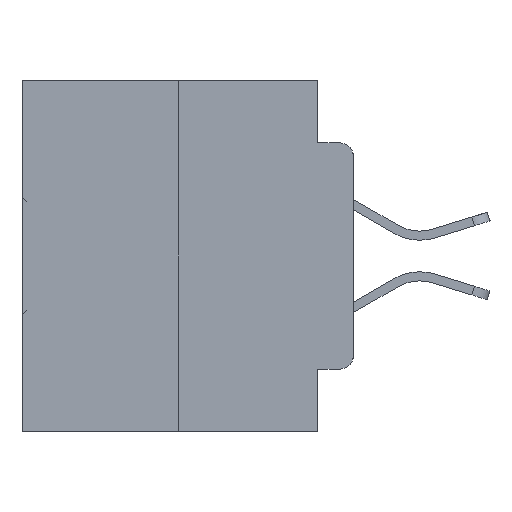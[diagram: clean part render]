
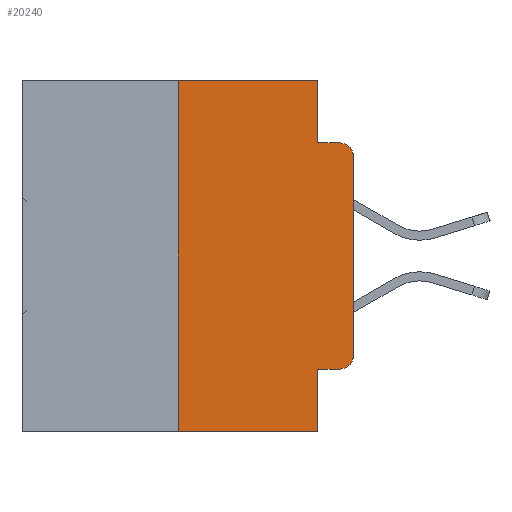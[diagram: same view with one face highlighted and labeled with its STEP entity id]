
A CAD part, left-side view. The second image highlights one B-rep face of the part: STEP entity #20240.
In plain terms, the highlighted planar face has unit normal (-1, 0, 0).
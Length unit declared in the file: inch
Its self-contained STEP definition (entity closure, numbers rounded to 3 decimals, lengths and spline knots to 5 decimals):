
#207 = EDGE_CURVE ( 'NONE', #18751, #5665, #8600, .T. ) ;
#492 = CARTESIAN_POINT ( 'NONE',  ( 0., 0.051, 0. ) ) ;
#687 = CARTESIAN_POINT ( 'NONE',  ( 0., 0.02, -0.4115 ) ) ;
#1872 = CARTESIAN_POINT ( 'NONE',  ( 0., 0.051, 0. ) ) ;
#2226 = CARTESIAN_POINT ( 'NONE',  ( 0., 0.051, -0.5 ) ) ;
#2351 = LINE ( 'NONE', #10271, #21443 ) ;
#2475 = CARTESIAN_POINT ( 'NONE',  ( 0., 0.473, -0.5 ) ) ;
#2622 = AXIS2_PLACEMENT_3D ( 'NONE', #25559, #23217, #22885 ) ;
#2670 = FACE_OUTER_BOUND ( 'NONE', #24543, .T. ) ;
#3357 = ORIENTED_EDGE ( 'NONE', *, *, #25172, .T. ) ;
#3578 = CARTESIAN_POINT ( 'NONE',  ( 0., 0.02, -0.0885 ) ) ;
#4313 = VERTEX_POINT ( 'NONE', #28794 ) ;
#4670 = LINE ( 'NONE', #2475, #7825 ) ;
#4744 = DIRECTION ( 'NONE',  ( 0., 0., -1. ) ) ;
#5144 = VECTOR ( 'NONE', #4744, 39.37008 ) ;
#5547 = ORIENTED_EDGE ( 'NONE', *, *, #18010, .F. ) ;
#5665 = VERTEX_POINT ( 'NONE', #19399 ) ;
#6133 = ORIENTED_EDGE ( 'NONE', *, *, #15103, .F. ) ;
#7130 = DIRECTION ( 'NONE',  ( 0., 0., 1. ) ) ;
#7234 = EDGE_CURVE ( 'NONE', #31207, #4313, #7448, .T. ) ;
#7403 = ORIENTED_EDGE ( 'NONE', *, *, #30107, .T. ) ;
#7448 = CIRCLE ( 'NONE', #13898, 0.02 ) ;
#7552 = DIRECTION ( 'NONE',  ( 0., -1., 0. ) ) ;
#7616 = LINE ( 'NONE', #1872, #5144 ) ;
#7628 = LINE ( 'NONE', #18245, #24825 ) ;
#7746 = EDGE_CURVE ( 'NONE', #26955, #31207, #24942, .T. ) ;
#7825 = VECTOR ( 'NONE', #7552, 39.37008 ) ;
#8117 = DIRECTION ( 'NONE',  ( 0., 0., -1. ) ) ;
#8600 = LINE ( 'NONE', #492, #26900 ) ;
#10271 = CARTESIAN_POINT ( 'NONE',  ( 0., 0.473, 0. ) ) ;
#11434 = VECTOR ( 'NONE', #11779, 39.37008 ) ;
#11779 = DIRECTION ( 'NONE',  ( 0., -1., 0. ) ) ;
#11863 = ORIENTED_EDGE ( 'NONE', *, *, #27198, .F. ) ;
#12675 = DIRECTION ( 'NONE',  ( -1., 0., 0. ) ) ;
#13898 = AXIS2_PLACEMENT_3D ( 'NONE', #17749, #12675, #8117 ) ;
#14205 = CARTESIAN_POINT ( 'NONE',  ( 0., 0.051, 0. ) ) ;
#14798 = CIRCLE ( 'NONE', #22863, 0.02 ) ;
#14809 = CARTESIAN_POINT ( 'NONE',  ( 0., 0.051, -0.0885 ) ) ;
#15103 = EDGE_CURVE ( 'NONE', #26955, #24203, #7616, .T. ) ;
#16980 = VERTEX_POINT ( 'NONE', #22307 ) ;
#17173 = LINE ( 'NONE', #14809, #11434 ) ;
#17567 = CARTESIAN_POINT ( 'NONE',  ( 0., 0.051, -0.4115 ) ) ;
#17598 = EDGE_CURVE ( 'NONE', #32058, #23787, #20089, .T. ) ;
#17749 = CARTESIAN_POINT ( 'NONE',  ( 0., 0.02, -0.3915 ) ) ;
#18010 = EDGE_CURVE ( 'NONE', #23787, #18751, #2351, .T. ) ;
#18214 = CARTESIAN_POINT ( 'NONE',  ( 0., 0.051, -0.4115 ) ) ;
#18245 = CARTESIAN_POINT ( 'NONE',  ( 0., 0., 0. ) ) ;
#18299 = CARTESIAN_POINT ( 'NONE',  ( 0., 0.25, -0.5 ) ) ;
#18543 = DIRECTION ( 'NONE',  ( 0., 0., -1. ) ) ;
#18751 = VERTEX_POINT ( 'NONE', #14205 ) ;
#18830 = DIRECTION ( 'NONE',  ( -1., 0., 0. ) ) ;
#19001 = ORIENTED_EDGE ( 'NONE', *, *, #17598, .F. ) ;
#19002 = DIRECTION ( 'NONE',  ( 0., 0., -1. ) ) ;
#19399 = CARTESIAN_POINT ( 'NONE',  ( 0., 0.051, -0.0885 ) ) ;
#20089 = LINE ( 'NONE', #30697, #20876 ) ;
#20240 = ADVANCED_FACE ( 'NONE', ( #2670 ), #22723, .F. ) ;
#20586 = DIRECTION ( 'NONE',  ( 0., 0., 1. ) ) ;
#20876 = VECTOR ( 'NONE', #7130, 39.37008 ) ;
#21443 = VECTOR ( 'NONE', #30661, 39.37008 ) ;
#21473 = VERTEX_POINT ( 'NONE', #3578 ) ;
#21668 = CARTESIAN_POINT ( 'NONE',  ( 0., 0.02, -0.1085 ) ) ;
#22307 = CARTESIAN_POINT ( 'NONE',  ( 0., 0., -0.1085 ) ) ;
#22421 = DIRECTION ( 'NONE',  ( 0., -1., 0. ) ) ;
#22654 = CARTESIAN_POINT ( 'NONE',  ( 0., 0.25, 0. ) ) ;
#22723 = PLANE ( 'NONE',  #2622 ) ;
#22863 = AXIS2_PLACEMENT_3D ( 'NONE', #21668, #18830, #19002 ) ;
#22885 = DIRECTION ( 'NONE',  ( 0., 0., -1. ) ) ;
#23217 = DIRECTION ( 'NONE',  ( 1., 0., 0. ) ) ;
#23787 = VERTEX_POINT ( 'NONE', #22654 ) ;
#24203 = VERTEX_POINT ( 'NONE', #2226 ) ;
#24543 = EDGE_LOOP ( 'NONE', ( #3357, #24856, #11863, #28618, #5547, #19001, #7403, #6133, #25002, #29573 ) ) ;
#24825 = VECTOR ( 'NONE', #20586, 39.37008 ) ;
#24856 = ORIENTED_EDGE ( 'NONE', *, *, #31567, .T. ) ;
#24942 = LINE ( 'NONE', #17567, #33291 ) ;
#25002 = ORIENTED_EDGE ( 'NONE', *, *, #7746, .T. ) ;
#25172 = EDGE_CURVE ( 'NONE', #4313, #16980, #7628, .T. ) ;
#25559 = CARTESIAN_POINT ( 'NONE',  ( 0., 0.473, 0. ) ) ;
#26900 = VECTOR ( 'NONE', #18543, 39.37008 ) ;
#26955 = VERTEX_POINT ( 'NONE', #18214 ) ;
#27198 = EDGE_CURVE ( 'NONE', #5665, #21473, #17173, .T. ) ;
#28618 = ORIENTED_EDGE ( 'NONE', *, *, #207, .F. ) ;
#28794 = CARTESIAN_POINT ( 'NONE',  ( 0., 0., -0.3915 ) ) ;
#29573 = ORIENTED_EDGE ( 'NONE', *, *, #7234, .T. ) ;
#30107 = EDGE_CURVE ( 'NONE', #32058, #24203, #4670, .T. ) ;
#30661 = DIRECTION ( 'NONE',  ( 0., -1., 0. ) ) ;
#30697 = CARTESIAN_POINT ( 'NONE',  ( 0., 0.25, 0. ) ) ;
#31207 = VERTEX_POINT ( 'NONE', #687 ) ;
#31567 = EDGE_CURVE ( 'NONE', #16980, #21473, #14798, .T. ) ;
#32058 = VERTEX_POINT ( 'NONE', #18299 ) ;
#33291 = VECTOR ( 'NONE', #22421, 39.37008 ) ;
